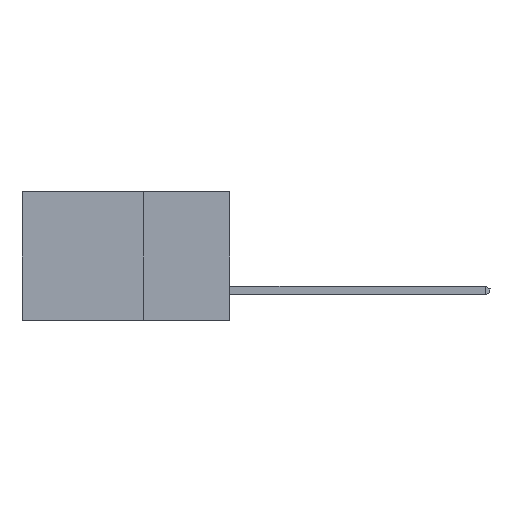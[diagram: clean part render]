
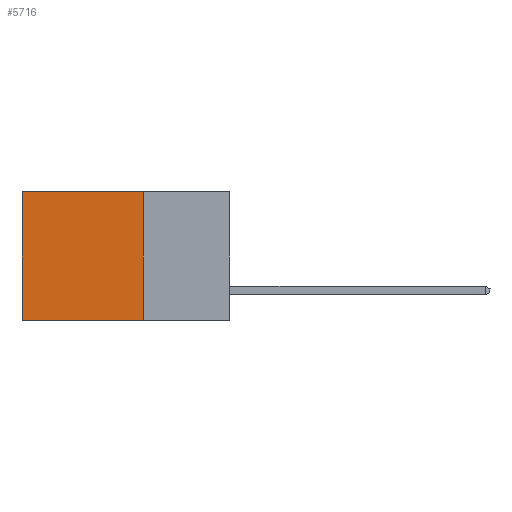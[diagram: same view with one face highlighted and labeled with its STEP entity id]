
A CAD part, left-side view. The second image highlights one B-rep face of the part: STEP entity #5716.
In plain terms, the highlighted planar face has unit normal (-1, 0, 0).
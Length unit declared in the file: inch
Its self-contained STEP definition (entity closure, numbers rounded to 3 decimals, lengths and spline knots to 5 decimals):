
#8 = CARTESIAN_POINT ( 'NONE',  ( 0.2615, 0.6, -0.37 ) ) ;
#21 = DIRECTION ( 'NONE',  ( 0., 1., 0. ) ) ;
#1234 = ORIENTED_EDGE ( 'NONE', *, *, #9056, .T. ) ;
#1981 = LINE ( 'NONE', #17998, #16844 ) ;
#2093 = CARTESIAN_POINT ( 'NONE',  ( 0.2615, 0.6, 0. ) ) ;
#3652 = DIRECTION ( 'NONE',  ( 0., 0., -1. ) ) ;
#3862 = EDGE_LOOP ( 'NONE', ( #1234, #9213, #9542, #7590 ) ) ;
#4620 = CARTESIAN_POINT ( 'NONE',  ( 0.2615, 0.25, 0. ) ) ;
#4795 = DIRECTION ( 'NONE',  ( 0., 1., 0. ) ) ;
#4995 = PLANE ( 'NONE',  #6204 ) ;
#5716 = ADVANCED_FACE ( 'NONE', ( #9619 ), #4995, .F. ) ;
#5783 = EDGE_CURVE ( 'NONE', #17637, #16582, #19150, .T. ) ;
#6102 = VERTEX_POINT ( 'NONE', #7392 ) ;
#6204 = AXIS2_PLACEMENT_3D ( 'NONE', #16235, #6670, #14664 ) ;
#6465 = CARTESIAN_POINT ( 'NONE',  ( 0.2615, 0.25, 0. ) ) ;
#6670 = DIRECTION ( 'NONE',  ( 1., 0., 0. ) ) ;
#7027 = VERTEX_POINT ( 'NONE', #8 ) ;
#7392 = CARTESIAN_POINT ( 'NONE',  ( 0.2615, 0.25, -0.37 ) ) ;
#7590 = ORIENTED_EDGE ( 'NONE', *, *, #5783, .T. ) ;
#7761 = LINE ( 'NONE', #14169, #19248 ) ;
#9056 = EDGE_CURVE ( 'NONE', #16582, #7027, #1981, .T. ) ;
#9213 = ORIENTED_EDGE ( 'NONE', *, *, #19984, .F. ) ;
#9542 = ORIENTED_EDGE ( 'NONE', *, *, #11426, .F. ) ;
#9619 = FACE_OUTER_BOUND ( 'NONE', #3862, .T. ) ;
#11426 = EDGE_CURVE ( 'NONE', #17637, #6102, #19955, .T. ) ;
#13680 = CARTESIAN_POINT ( 'NONE',  ( 0.2615, 0.25, -0.37 ) ) ;
#14169 = CARTESIAN_POINT ( 'NONE',  ( 0.2615, 0.25, -0.37 ) ) ;
#14664 = DIRECTION ( 'NONE',  ( 0., 0., -1. ) ) ;
#15265 = DIRECTION ( 'NONE',  ( 0., 0., -1. ) ) ;
#16235 = CARTESIAN_POINT ( 'NONE',  ( 0.2615, 0.25, -0.37 ) ) ;
#16582 = VERTEX_POINT ( 'NONE', #2093 ) ;
#16844 = VECTOR ( 'NONE', #3652, 39.37008 ) ;
#17637 = VERTEX_POINT ( 'NONE', #4620 ) ;
#17998 = CARTESIAN_POINT ( 'NONE',  ( 0.2615, 0.6, -0.37 ) ) ;
#18591 = VECTOR ( 'NONE', #15265, 39.37008 ) ;
#18926 = VECTOR ( 'NONE', #4795, 39.37008 ) ;
#19150 = LINE ( 'NONE', #6465, #18926 ) ;
#19248 = VECTOR ( 'NONE', #21, 39.37008 ) ;
#19955 = LINE ( 'NONE', #13680, #18591 ) ;
#19984 = EDGE_CURVE ( 'NONE', #6102, #7027, #7761, .T. ) ;
